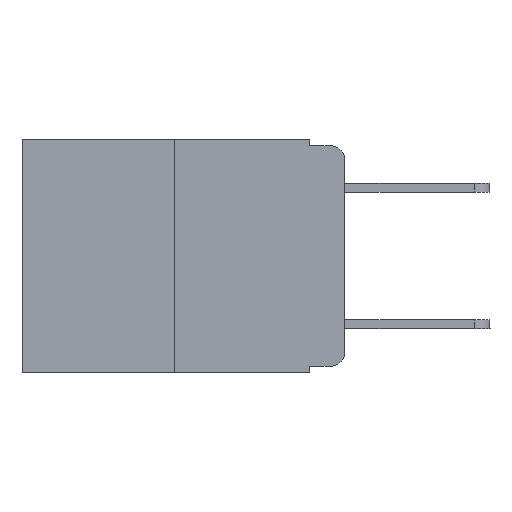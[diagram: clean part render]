
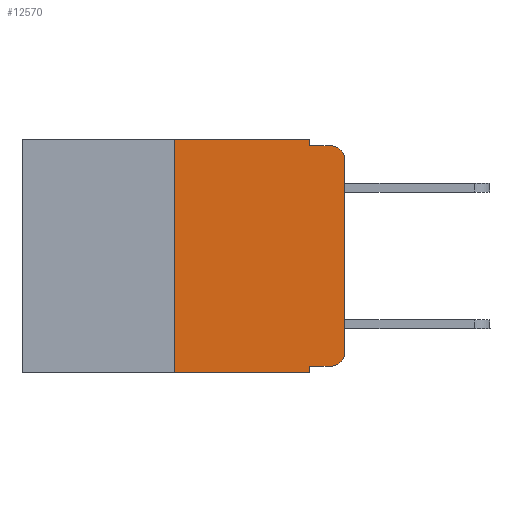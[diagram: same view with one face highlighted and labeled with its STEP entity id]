
A CAD part, left-side view. The second image highlights one B-rep face of the part: STEP entity #12570.
In plain terms, the highlighted planar face has unit normal (-1, 0, 0).
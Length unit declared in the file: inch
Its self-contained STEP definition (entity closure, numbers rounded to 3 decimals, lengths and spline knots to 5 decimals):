
#4 = VERTEX_POINT ( 'NONE', #2828 ) ;
#53 = CARTESIAN_POINT ( 'NONE',  ( 0., 0., -0.313 ) ) ;
#60 = AXIS2_PLACEMENT_3D ( 'NONE', #4612, #3507, #5834 ) ;
#296 = EDGE_CURVE ( 'NONE', #4, #10940, #3474, .T. ) ;
#317 = LINE ( 'NONE', #4872, #11027 ) ;
#393 = DIRECTION ( 'NONE',  ( 0., -1., 0. ) ) ;
#501 = VECTOR ( 'NONE', #9971, 39.37008 ) ;
#540 = CARTESIAN_POINT ( 'NONE',  ( 0., 0.473, 0. ) ) ;
#670 = CARTESIAN_POINT ( 'NONE',  ( 0., 0.473, -0.343 ) ) ;
#734 = ORIENTED_EDGE ( 'NONE', *, *, #2965, .F. ) ;
#871 = CARTESIAN_POINT ( 'NONE',  ( 0., 0.051, 0. ) ) ;
#939 = EDGE_CURVE ( 'NONE', #8460, #14282, #5974, .T. ) ;
#1733 = LINE ( 'NONE', #540, #13060 ) ;
#2616 = CARTESIAN_POINT ( 'NONE',  ( 0., 0.02, -0.01 ) ) ;
#2828 = CARTESIAN_POINT ( 'NONE',  ( 0., 0.051, -0.01 ) ) ;
#2965 = EDGE_CURVE ( 'NONE', #14103, #14175, #1733, .T. ) ;
#3169 = CIRCLE ( 'NONE', #10332, 0.02 ) ;
#3207 = ORIENTED_EDGE ( 'NONE', *, *, #9295, .F. ) ;
#3474 = LINE ( 'NONE', #8062, #9156 ) ;
#3507 = DIRECTION ( 'NONE',  ( 1., 0., 0. ) ) ;
#3706 = VERTEX_POINT ( 'NONE', #11563 ) ;
#3717 = EDGE_LOOP ( 'NONE', ( #4654, #8695, #8573, #3207, #734, #6659, #12900, #8847, #4828, #5377 ) ) ;
#4083 = EDGE_CURVE ( 'NONE', #7682, #8460, #7753, .T. ) ;
#4500 = VECTOR ( 'NONE', #5239, 39.37008 ) ;
#4612 = CARTESIAN_POINT ( 'NONE',  ( 0., 0.473, 0. ) ) ;
#4654 = ORIENTED_EDGE ( 'NONE', *, *, #9430, .T. ) ;
#4692 = FACE_OUTER_BOUND ( 'NONE', #3717, .T. ) ;
#4828 = ORIENTED_EDGE ( 'NONE', *, *, #4083, .T. ) ;
#4872 = CARTESIAN_POINT ( 'NONE',  ( 0., 0., 0. ) ) ;
#5140 = DIRECTION ( 'NONE',  ( 0., 0., -1. ) ) ;
#5239 = DIRECTION ( 'NONE',  ( 0., -1., 0. ) ) ;
#5377 = ORIENTED_EDGE ( 'NONE', *, *, #939, .T. ) ;
#5541 = DIRECTION ( 'NONE',  ( -1., 0., 0. ) ) ;
#5834 = DIRECTION ( 'NONE',  ( 0., 0., -1. ) ) ;
#5974 = CIRCLE ( 'NONE', #14333, 0.02 ) ;
#5992 = EDGE_CURVE ( 'NONE', #13379, #7552, #7572, .T. ) ;
#6328 = EDGE_CURVE ( 'NONE', #7682, #7552, #12090, .T. ) ;
#6401 = VECTOR ( 'NONE', #13706, 39.37008 ) ;
#6659 = ORIENTED_EDGE ( 'NONE', *, *, #12802, .F. ) ;
#6929 = DIRECTION ( 'NONE',  ( 0., -1., 0. ) ) ;
#7113 = CARTESIAN_POINT ( 'NONE',  ( 0., 0.02, -0.333 ) ) ;
#7279 = CARTESIAN_POINT ( 'NONE',  ( 0., 0.02, -0.313 ) ) ;
#7552 = VERTEX_POINT ( 'NONE', #7834 ) ;
#7572 = LINE ( 'NONE', #670, #4500 ) ;
#7682 = VERTEX_POINT ( 'NONE', #13717 ) ;
#7753 = LINE ( 'NONE', #10049, #6401 ) ;
#7834 = CARTESIAN_POINT ( 'NONE',  ( 0., 0.051, -0.343 ) ) ;
#8062 = CARTESIAN_POINT ( 'NONE',  ( 0., 0.051, -0.01 ) ) ;
#8092 = PLANE ( 'NONE',  #60 ) ;
#8460 = VERTEX_POINT ( 'NONE', #7113 ) ;
#8573 = ORIENTED_EDGE ( 'NONE', *, *, #296, .F. ) ;
#8613 = CARTESIAN_POINT ( 'NONE',  ( 0., 0.02, -0.03 ) ) ;
#8695 = ORIENTED_EDGE ( 'NONE', *, *, #11118, .T. ) ;
#8847 = ORIENTED_EDGE ( 'NONE', *, *, #6328, .F. ) ;
#9156 = VECTOR ( 'NONE', #6929, 39.37008 ) ;
#9162 = CARTESIAN_POINT ( 'NONE',  ( 0., 0.051, 0. ) ) ;
#9295 = EDGE_CURVE ( 'NONE', #14175, #4, #12510, .T. ) ;
#9430 = EDGE_CURVE ( 'NONE', #14282, #3706, #317, .T. ) ;
#9459 = DIRECTION ( 'NONE',  ( 0., 0., 1. ) ) ;
#9971 = DIRECTION ( 'NONE',  ( 0., 0., -1. ) ) ;
#10049 = CARTESIAN_POINT ( 'NONE',  ( 0., 0.051, -0.333 ) ) ;
#10332 = AXIS2_PLACEMENT_3D ( 'NONE', #8613, #13066, #14341 ) ;
#10940 = VERTEX_POINT ( 'NONE', #2616 ) ;
#10953 = VECTOR ( 'NONE', #5140, 39.37008 ) ;
#11027 = VECTOR ( 'NONE', #9459, 39.37008 ) ;
#11118 = EDGE_CURVE ( 'NONE', #3706, #10940, #3169, .T. ) ;
#11383 = CARTESIAN_POINT ( 'NONE',  ( 0., 0.25, -0.343 ) ) ;
#11563 = CARTESIAN_POINT ( 'NONE',  ( 0., 0., -0.03 ) ) ;
#11807 = DIRECTION ( 'NONE',  ( 0., 0., 1. ) ) ;
#12090 = LINE ( 'NONE', #13136, #10953 ) ;
#12510 = LINE ( 'NONE', #9162, #501 ) ;
#12570 = ADVANCED_FACE ( 'NONE', ( #4692 ), #8092, .F. ) ;
#12802 = EDGE_CURVE ( 'NONE', #13379, #14103, #13977, .T. ) ;
#12900 = ORIENTED_EDGE ( 'NONE', *, *, #5992, .T. ) ;
#12967 = VECTOR ( 'NONE', #11807, 39.37008 ) ;
#12999 = CARTESIAN_POINT ( 'NONE',  ( 0., 0.25, 0. ) ) ;
#13060 = VECTOR ( 'NONE', #393, 39.37008 ) ;
#13066 = DIRECTION ( 'NONE',  ( -1., 0., 0. ) ) ;
#13136 = CARTESIAN_POINT ( 'NONE',  ( 0., 0.051, 0. ) ) ;
#13379 = VERTEX_POINT ( 'NONE', #11383 ) ;
#13706 = DIRECTION ( 'NONE',  ( 0., -1., 0. ) ) ;
#13717 = CARTESIAN_POINT ( 'NONE',  ( 0., 0.051, -0.333 ) ) ;
#13977 = LINE ( 'NONE', #14194, #12967 ) ;
#14103 = VERTEX_POINT ( 'NONE', #12999 ) ;
#14175 = VERTEX_POINT ( 'NONE', #871 ) ;
#14194 = CARTESIAN_POINT ( 'NONE',  ( 0., 0.25, 0. ) ) ;
#14282 = VERTEX_POINT ( 'NONE', #53 ) ;
#14333 = AXIS2_PLACEMENT_3D ( 'NONE', #7279, #5541, #14432 ) ;
#14341 = DIRECTION ( 'NONE',  ( 0., 0., -1. ) ) ;
#14432 = DIRECTION ( 'NONE',  ( 0., 0., -1. ) ) ;
